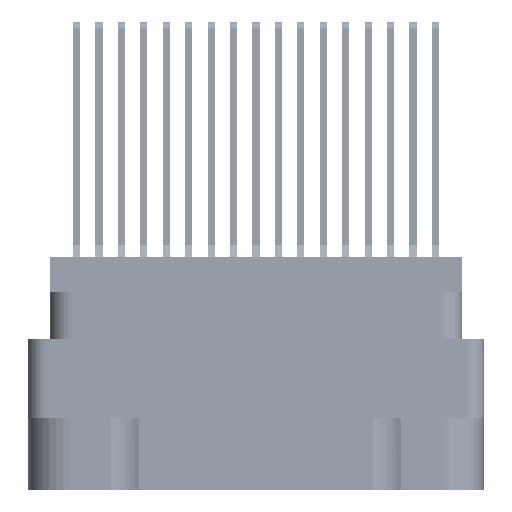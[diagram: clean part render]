
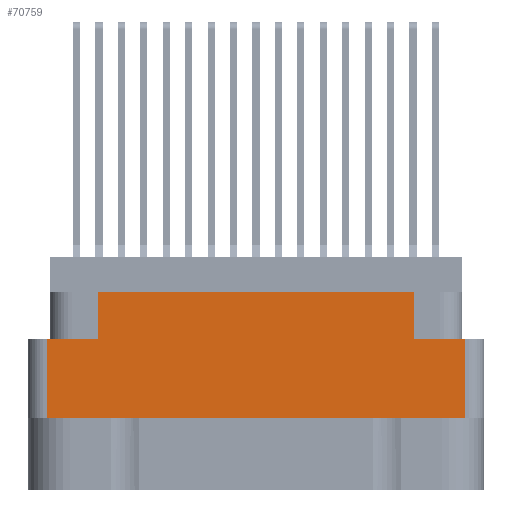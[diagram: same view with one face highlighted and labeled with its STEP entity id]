
A CAD part, left-side view. The second image highlights one B-rep face of the part: STEP entity #70759.
In plain terms, the highlighted planar face has unit normal (-1, 0, 0).
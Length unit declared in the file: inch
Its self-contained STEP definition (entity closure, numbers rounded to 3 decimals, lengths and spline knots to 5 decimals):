
#542 = DIRECTION ( 'NONE',  ( 0., 0., 1. ) ) ;
#4086 = DIRECTION ( 'NONE',  ( 0., 0., 1. ) ) ;
#4872 = CARTESIAN_POINT ( 'NONE',  ( -1.375, 0.7005, -0.78 ) ) ;
#6669 = DIRECTION ( 'NONE',  ( -1., 0., 0. ) ) ;
#8165 = VECTOR ( 'NONE', #73849, 39.37008 ) ;
#11646 = CARTESIAN_POINT ( 'NONE',  ( -1.375, -0.7005, -0.54 ) ) ;
#13142 = LINE ( 'NONE', #86710, #75395 ) ;
#14738 = LINE ( 'NONE', #38762, #8165 ) ;
#14911 = DIRECTION ( 'NONE',  ( 0., -1., 0. ) ) ;
#17136 = DIRECTION ( 'NONE',  ( 0., -1., 0. ) ) ;
#17389 = VERTEX_POINT ( 'NONE', #63626 ) ;
#17998 = EDGE_LOOP ( 'NONE', ( #86904, #42900, #58790, #76147, #43653, #79225, #78823, #19979 ) ) ;
#18852 = CARTESIAN_POINT ( 'NONE',  ( -1.375, -0.5285, -0.274 ) ) ;
#19156 = VERTEX_POINT ( 'NONE', #43817 ) ;
#19979 = ORIENTED_EDGE ( 'NONE', *, *, #72333, .F. ) ;
#24832 = DIRECTION ( 'NONE',  ( 0., 0., 1. ) ) ;
#24941 = DIRECTION ( 'NONE',  ( 0., 0., 1. ) ) ;
#25269 = LINE ( 'NONE', #18852, #55782 ) ;
#25559 = LINE ( 'NONE', #70744, #27766 ) ;
#27073 = EDGE_CURVE ( 'NONE', #79480, #76478, #25559, .T. ) ;
#27766 = VECTOR ( 'NONE', #14911, 39.37008 ) ;
#28090 = EDGE_CURVE ( 'NONE', #35076, #19156, #67948, .T. ) ;
#32346 = DIRECTION ( 'NONE',  ( 0., 0., -1. ) ) ;
#35076 = VERTEX_POINT ( 'NONE', #11646 ) ;
#35618 = CARTESIAN_POINT ( 'NONE',  ( -1.375, 0.7005, -0.274 ) ) ;
#35709 = VERTEX_POINT ( 'NONE', #68008 ) ;
#36528 = VECTOR ( 'NONE', #87144, 39.37008 ) ;
#37323 = LINE ( 'NONE', #4872, #74460 ) ;
#37625 = CARTESIAN_POINT ( 'NONE',  ( -1.375, 0.5285, -0.274 ) ) ;
#38762 = CARTESIAN_POINT ( 'NONE',  ( -1.375, 0., -0.54 ) ) ;
#39575 = VECTOR ( 'NONE', #4086, 39.37008 ) ;
#40558 = EDGE_CURVE ( 'NONE', #79480, #41847, #37323, .T. ) ;
#41847 = VERTEX_POINT ( 'NONE', #52828 ) ;
#42900 = ORIENTED_EDGE ( 'NONE', *, *, #40558, .T. ) ;
#43653 = ORIENTED_EDGE ( 'NONE', *, *, #59176, .F. ) ;
#43817 = CARTESIAN_POINT ( 'NONE',  ( -1.375, -0.7005, -0.274 ) ) ;
#45564 = CARTESIAN_POINT ( 'NONE',  ( -1.375, -0.7005, -0.78 ) ) ;
#46145 = EDGE_CURVE ( 'NONE', #75023, #17389, #25269, .T. ) ;
#50942 = EDGE_CURVE ( 'NONE', #41847, #35076, #14738, .T. ) ;
#52828 = CARTESIAN_POINT ( 'NONE',  ( -1.375, 0.7005, -0.54 ) ) ;
#55622 = EDGE_CURVE ( 'NONE', #35709, #17389, #84632, .T. ) ;
#55782 = VECTOR ( 'NONE', #24941, 39.37008 ) ;
#56307 = PLANE ( 'NONE',  #64672 ) ;
#56606 = CARTESIAN_POINT ( 'NONE',  ( -1.375, -0.7625, -0.78 ) ) ;
#58660 = CARTESIAN_POINT ( 'NONE',  ( -1.375, 0.5285, -0.274 ) ) ;
#58790 = ORIENTED_EDGE ( 'NONE', *, *, #50942, .T. ) ;
#59176 = EDGE_CURVE ( 'NONE', #75023, #19156, #13142, .T. ) ;
#62114 = VECTOR ( 'NONE', #24832, 39.37008 ) ;
#63299 = CARTESIAN_POINT ( 'NONE',  ( -1.375, -0.5285, -0.274 ) ) ;
#63626 = CARTESIAN_POINT ( 'NONE',  ( -1.375, -0.5285, -0.117 ) ) ;
#64672 = AXIS2_PLACEMENT_3D ( 'NONE', #56606, #6669, #542 ) ;
#67948 = LINE ( 'NONE', #45564, #39575 ) ;
#68008 = CARTESIAN_POINT ( 'NONE',  ( -1.375, 0.5285, -0.117 ) ) ;
#70744 = CARTESIAN_POINT ( 'NONE',  ( -1.375, 0., -0.274 ) ) ;
#70759 = ADVANCED_FACE ( 'NONE', ( #86377 ), #56307, .T. ) ;
#72333 = EDGE_CURVE ( 'NONE', #76478, #35709, #89521, .T. ) ;
#73849 = DIRECTION ( 'NONE',  ( 0., -1., 0. ) ) ;
#74460 = VECTOR ( 'NONE', #32346, 39.37008 ) ;
#75023 = VERTEX_POINT ( 'NONE', #63299 ) ;
#75395 = VECTOR ( 'NONE', #17136, 39.37008 ) ;
#75877 = CARTESIAN_POINT ( 'NONE',  ( -1.375, 0.7625, -0.117 ) ) ;
#76147 = ORIENTED_EDGE ( 'NONE', *, *, #28090, .T. ) ;
#76478 = VERTEX_POINT ( 'NONE', #37625 ) ;
#78823 = ORIENTED_EDGE ( 'NONE', *, *, #55622, .F. ) ;
#79225 = ORIENTED_EDGE ( 'NONE', *, *, #46145, .T. ) ;
#79480 = VERTEX_POINT ( 'NONE', #35618 ) ;
#84632 = LINE ( 'NONE', #75877, #36528 ) ;
#86377 = FACE_OUTER_BOUND ( 'NONE', #17998, .T. ) ;
#86710 = CARTESIAN_POINT ( 'NONE',  ( -1.375, 0., -0.274 ) ) ;
#86904 = ORIENTED_EDGE ( 'NONE', *, *, #27073, .F. ) ;
#87144 = DIRECTION ( 'NONE',  ( 0., -1., 0. ) ) ;
#89521 = LINE ( 'NONE', #58660, #62114 ) ;
